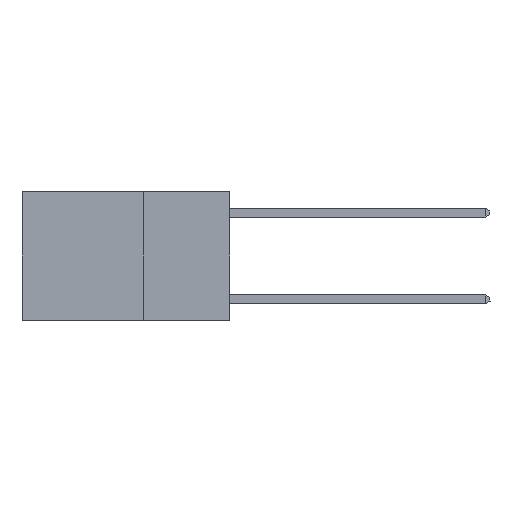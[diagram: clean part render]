
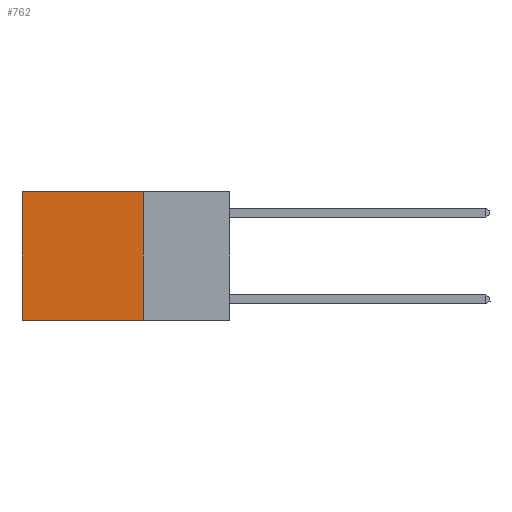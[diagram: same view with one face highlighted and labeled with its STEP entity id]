
A CAD part, left-side view. The second image highlights one B-rep face of the part: STEP entity #762.
In plain terms, the highlighted planar face has unit normal (-1, 0, 0).
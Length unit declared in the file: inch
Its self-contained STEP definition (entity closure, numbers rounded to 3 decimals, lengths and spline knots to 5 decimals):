
#762 = ADVANCED_FACE ( 'NONE', ( #8582 ), #17589, .F. ) ;
#888 = CARTESIAN_POINT ( 'NONE',  ( 0.2625, 0.6, -0.37 ) ) ;
#1546 = DIRECTION ( 'NONE',  ( 0., 0., -1. ) ) ;
#2547 = DIRECTION ( 'NONE',  ( 0., 0., -1. ) ) ;
#2744 = CARTESIAN_POINT ( 'NONE',  ( 0.2625, 0.25, 0. ) ) ;
#5530 = CARTESIAN_POINT ( 'NONE',  ( 0.2625, 0.25, -0.37 ) ) ;
#5662 = ORIENTED_EDGE ( 'NONE', *, *, #17787, .F. ) ;
#6262 = CARTESIAN_POINT ( 'NONE',  ( 0.2625, 0.25, 0. ) ) ;
#8582 = FACE_OUTER_BOUND ( 'NONE', #24364, .T. ) ;
#8759 = ORIENTED_EDGE ( 'NONE', *, *, #14789, .T. ) ;
#9037 = DIRECTION ( 'NONE',  ( 0., 0., -1. ) ) ;
#9437 = VECTOR ( 'NONE', #17690, 39.37008 ) ;
#10144 = LINE ( 'NONE', #16525, #25841 ) ;
#10532 = ORIENTED_EDGE ( 'NONE', *, *, #18708, .T. ) ;
#11100 = CARTESIAN_POINT ( 'NONE',  ( 0.2625, 0.25, 0. ) ) ;
#13673 = VECTOR ( 'NONE', #18353, 39.37008 ) ;
#14789 = EDGE_CURVE ( 'NONE', #24173, #17516, #16004, .T. ) ;
#15896 = VERTEX_POINT ( 'NONE', #6262 ) ;
#16004 = LINE ( 'NONE', #19651, #26611 ) ;
#16525 = CARTESIAN_POINT ( 'NONE',  ( 0.2625, 0.25, 0. ) ) ;
#17516 = VERTEX_POINT ( 'NONE', #888 ) ;
#17589 = PLANE ( 'NONE',  #20816 ) ;
#17690 = DIRECTION ( 'NONE',  ( 0., 1., 0. ) ) ;
#17787 = EDGE_CURVE ( 'NONE', #15896, #21349, #10144, .T. ) ;
#18353 = DIRECTION ( 'NONE',  ( 0., 1., 0. ) ) ;
#18708 = EDGE_CURVE ( 'NONE', #15896, #24173, #20855, .T. ) ;
#19651 = CARTESIAN_POINT ( 'NONE',  ( 0.2625, 0.6, 0. ) ) ;
#20816 = AXIS2_PLACEMENT_3D ( 'NONE', #11100, #21893, #9037 ) ;
#20855 = LINE ( 'NONE', #2744, #9437 ) ;
#21349 = VERTEX_POINT ( 'NONE', #21903 ) ;
#21515 = CARTESIAN_POINT ( 'NONE',  ( 0.2625, 0.6, 0. ) ) ;
#21893 = DIRECTION ( 'NONE',  ( 1., 0., 0. ) ) ;
#21903 = CARTESIAN_POINT ( 'NONE',  ( 0.2625, 0.25, -0.37 ) ) ;
#23908 = EDGE_CURVE ( 'NONE', #21349, #17516, #25010, .T. ) ;
#24173 = VERTEX_POINT ( 'NONE', #21515 ) ;
#24364 = EDGE_LOOP ( 'NONE', ( #8759, #25273, #5662, #10532 ) ) ;
#25010 = LINE ( 'NONE', #5530, #13673 ) ;
#25273 = ORIENTED_EDGE ( 'NONE', *, *, #23908, .F. ) ;
#25841 = VECTOR ( 'NONE', #1546, 39.37008 ) ;
#26611 = VECTOR ( 'NONE', #2547, 39.37008 ) ;
